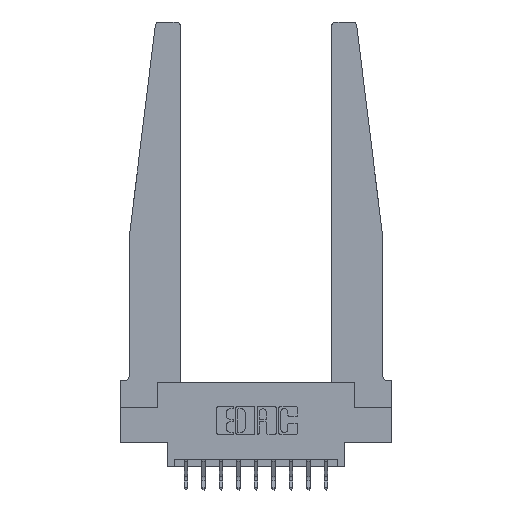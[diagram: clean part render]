
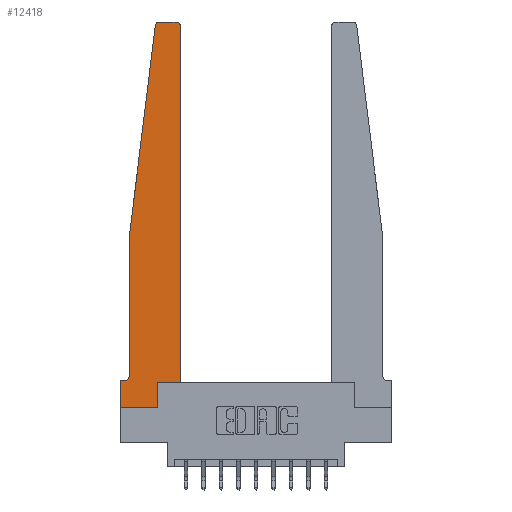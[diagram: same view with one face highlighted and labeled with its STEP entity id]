
A CAD part, top view. The second image highlights one B-rep face of the part: STEP entity #12418.
In plain terms, the highlighted planar face has unit normal (0, 0, 1).
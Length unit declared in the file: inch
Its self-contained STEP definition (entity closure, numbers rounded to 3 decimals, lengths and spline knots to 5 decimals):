
#168 = DIRECTION ( 'NONE',  ( 1., 0., 0. ) ) ;
#171 = CARTESIAN_POINT ( 'NONE',  ( 0.065, 0.2375, 0.37 ) ) ;
#614 = AXIS2_PLACEMENT_3D ( 'NONE', #6861, #12093, #15439 ) ;
#755 = VERTEX_POINT ( 'NONE', #2307 ) ;
#815 = VERTEX_POINT ( 'NONE', #12450 ) ;
#937 = VECTOR ( 'NONE', #14839, 39.37008 ) ;
#1153 = CARTESIAN_POINT ( 'NONE',  ( 0.24675, 2.72367, 0.37 ) ) ;
#1248 = CARTESIAN_POINT ( 'NONE',  ( 0.065, 1.25, 0.37 ) ) ;
#1255 = CARTESIAN_POINT ( 'NONE',  ( 0.065, 1.25, 0.37 ) ) ;
#1333 = LINE ( 'NONE', #1418, #3230 ) ;
#1418 = CARTESIAN_POINT ( 'NONE',  ( 0.425, 0.18, 0.37 ) ) ;
#1515 = CIRCLE ( 'NONE', #6381, 0.03 ) ;
#1588 = CARTESIAN_POINT ( 'NONE',  ( 0.425, 0.18, 0.37 ) ) ;
#1728 = CARTESIAN_POINT ( 'NONE',  ( 0.27653, 2.75, 0.37 ) ) ;
#1871 = VERTEX_POINT ( 'NONE', #1728 ) ;
#2116 = DIRECTION ( 'NONE',  ( 1., 0., 0. ) ) ;
#2224 = LINE ( 'NONE', #3509, #14038 ) ;
#2307 = CARTESIAN_POINT ( 'NONE',  ( 0.425, 2.72, 0.37 ) ) ;
#2387 = CIRCLE ( 'NONE', #8816, 0.05 ) ;
#3230 = VECTOR ( 'NONE', #11326, 39.37008 ) ;
#3509 = CARTESIAN_POINT ( 'NONE',  ( 0.25, 2.75, 0.37 ) ) ;
#3532 = LINE ( 'NONE', #4890, #6812 ) ;
#3568 = LINE ( 'NONE', #1248, #9054 ) ;
#3589 = ORIENTED_EDGE ( 'NONE', *, *, #12966, .T. ) ;
#4128 = EDGE_CURVE ( 'NONE', #14199, #14481, #10211, .T. ) ;
#4282 = AXIS2_PLACEMENT_3D ( 'NONE', #10113, #15089, #14853 ) ;
#4322 = EDGE_LOOP ( 'NONE', ( #15721, #4965, #4641, #14499, #8190, #3589, #13950, #9178, #8155, #10046, #14879, #13822 ) ) ;
#4424 = DIRECTION ( 'NONE',  ( 0., 0., -1. ) ) ;
#4627 = LINE ( 'NONE', #4708, #8871 ) ;
#4641 = ORIENTED_EDGE ( 'NONE', *, *, #6868, .T. ) ;
#4699 = LINE ( 'NONE', #7141, #937 ) ;
#4708 = CARTESIAN_POINT ( 'NONE',  ( 0., 0., 0.37 ) ) ;
#4890 = CARTESIAN_POINT ( 'NONE',  ( 0.065, 0.1875, 0.37 ) ) ;
#4965 = ORIENTED_EDGE ( 'NONE', *, *, #8324, .T. ) ;
#5220 = CARTESIAN_POINT ( 'NONE',  ( 0., 0.1875, 0.37 ) ) ;
#5680 = EDGE_CURVE ( 'NONE', #14481, #6093, #4627, .T. ) ;
#6093 = VERTEX_POINT ( 'NONE', #6160 ) ;
#6160 = CARTESIAN_POINT ( 'NONE',  ( 0.2605, 0., 0.37 ) ) ;
#6179 = VERTEX_POINT ( 'NONE', #1255 ) ;
#6381 = AXIS2_PLACEMENT_3D ( 'NONE', #9074, #10217, #168 ) ;
#6812 = VECTOR ( 'NONE', #7163, 39.37008 ) ;
#6861 = CARTESIAN_POINT ( 'NONE',  ( 0., 0.1875, 0.37 ) ) ;
#6868 = EDGE_CURVE ( 'NONE', #9339, #6179, #13291, .T. ) ;
#6893 = VERTEX_POINT ( 'NONE', #7424 ) ;
#7141 = CARTESIAN_POINT ( 'NONE',  ( 0.2605, 0.18, 0.37 ) ) ;
#7163 = DIRECTION ( 'NONE',  ( -1., 0., 0. ) ) ;
#7350 = EDGE_CURVE ( 'NONE', #755, #815, #13035, .T. ) ;
#7424 = CARTESIAN_POINT ( 'NONE',  ( 0.2605, 0.18, 0.37 ) ) ;
#7999 = CARTESIAN_POINT ( 'NONE',  ( 0., 0., 0.37 ) ) ;
#8155 = ORIENTED_EDGE ( 'NONE', *, *, #15365, .T. ) ;
#8190 = ORIENTED_EDGE ( 'NONE', *, *, #9552, .T. ) ;
#8312 = CARTESIAN_POINT ( 'NONE',  ( 0.425, 0.18, 0.37 ) ) ;
#8315 = DIRECTION ( 'NONE',  ( 0., -1., 0. ) ) ;
#8324 = EDGE_CURVE ( 'NONE', #1871, #9339, #1515, .T. ) ;
#8816 = AXIS2_PLACEMENT_3D ( 'NONE', #11934, #4424, #9270 ) ;
#8871 = VECTOR ( 'NONE', #9637, 39.37008 ) ;
#9054 = VECTOR ( 'NONE', #8315, 39.37008 ) ;
#9074 = CARTESIAN_POINT ( 'NONE',  ( 0.27653, 2.72, 0.37 ) ) ;
#9178 = ORIENTED_EDGE ( 'NONE', *, *, #5680, .T. ) ;
#9270 = DIRECTION ( 'NONE',  ( -1., 0., 0. ) ) ;
#9339 = VERTEX_POINT ( 'NONE', #1153 ) ;
#9552 = EDGE_CURVE ( 'NONE', #13396, #11178, #2387, .T. ) ;
#9637 = DIRECTION ( 'NONE',  ( 1., 0., 0. ) ) ;
#10046 = ORIENTED_EDGE ( 'NONE', *, *, #11977, .T. ) ;
#10113 = CARTESIAN_POINT ( 'NONE',  ( 0.395, 2.72, 0.37 ) ) ;
#10119 = VECTOR ( 'NONE', #2116, 39.37008 ) ;
#10148 = VERTEX_POINT ( 'NONE', #1588 ) ;
#10211 = LINE ( 'NONE', #13516, #12505 ) ;
#10217 = DIRECTION ( 'NONE',  ( 0., 0., 1. ) ) ;
#10731 = PLANE ( 'NONE',  #614 ) ;
#11178 = VERTEX_POINT ( 'NONE', #14320 ) ;
#11326 = DIRECTION ( 'NONE',  ( 0., 1., 0. ) ) ;
#11934 = CARTESIAN_POINT ( 'NONE',  ( 0.015, 0.2375, 0.37 ) ) ;
#11977 = EDGE_CURVE ( 'NONE', #6893, #10148, #14497, .T. ) ;
#12093 = DIRECTION ( 'NONE',  ( 0., 0., 1. ) ) ;
#12367 = DIRECTION ( 'NONE',  ( -1., 0., 0. ) ) ;
#12418 = ADVANCED_FACE ( 'NONE', ( #15673 ), #10731, .T. ) ;
#12450 = CARTESIAN_POINT ( 'NONE',  ( 0.395, 2.75, 0.37 ) ) ;
#12471 = DIRECTION ( 'NONE',  ( 0., -1., 0. ) ) ;
#12505 = VECTOR ( 'NONE', #12471, 39.37008 ) ;
#12966 = EDGE_CURVE ( 'NONE', #11178, #14199, #3532, .T. ) ;
#13035 = CIRCLE ( 'NONE', #4282, 0.03 ) ;
#13291 = LINE ( 'NONE', #14470, #15571 ) ;
#13396 = VERTEX_POINT ( 'NONE', #171 ) ;
#13516 = CARTESIAN_POINT ( 'NONE',  ( 0., 0., 0.37 ) ) ;
#13822 = ORIENTED_EDGE ( 'NONE', *, *, #7350, .T. ) ;
#13950 = ORIENTED_EDGE ( 'NONE', *, *, #4128, .T. ) ;
#14038 = VECTOR ( 'NONE', #12367, 39.37008 ) ;
#14199 = VERTEX_POINT ( 'NONE', #5220 ) ;
#14245 = EDGE_CURVE ( 'NONE', #10148, #755, #1333, .T. ) ;
#14320 = CARTESIAN_POINT ( 'NONE',  ( 0.015, 0.1875, 0.37 ) ) ;
#14470 = CARTESIAN_POINT ( 'NONE',  ( 0.065, 1.25, 0.37 ) ) ;
#14481 = VERTEX_POINT ( 'NONE', #7999 ) ;
#14497 = LINE ( 'NONE', #8312, #10119 ) ;
#14499 = ORIENTED_EDGE ( 'NONE', *, *, #15790, .T. ) ;
#14839 = DIRECTION ( 'NONE',  ( 0., 1., 0. ) ) ;
#14853 = DIRECTION ( 'NONE',  ( 1., 0., 0. ) ) ;
#14879 = ORIENTED_EDGE ( 'NONE', *, *, #14245, .T. ) ;
#15089 = DIRECTION ( 'NONE',  ( 0., 0., 1. ) ) ;
#15340 = EDGE_CURVE ( 'NONE', #815, #1871, #2224, .T. ) ;
#15365 = EDGE_CURVE ( 'NONE', #6093, #6893, #4699, .T. ) ;
#15439 = DIRECTION ( 'NONE',  ( 1., 0., 0. ) ) ;
#15571 = VECTOR ( 'NONE', #15842, 39.37008 ) ;
#15673 = FACE_OUTER_BOUND ( 'NONE', #4322, .T. ) ;
#15721 = ORIENTED_EDGE ( 'NONE', *, *, #15340, .T. ) ;
#15790 = EDGE_CURVE ( 'NONE', #6179, #13396, #3568, .T. ) ;
#15842 = DIRECTION ( 'NONE',  ( -0.122, -0.992, 0. ) ) ;
